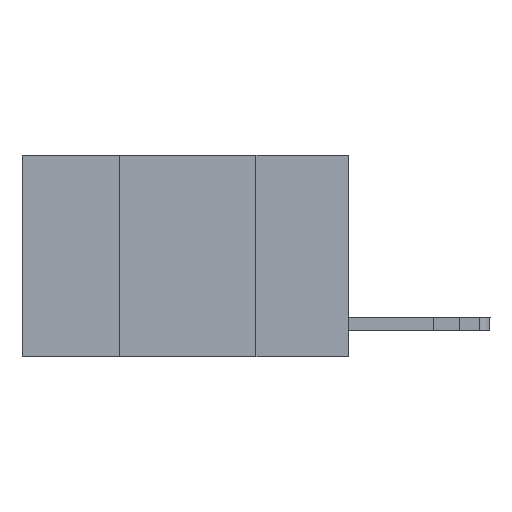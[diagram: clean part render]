
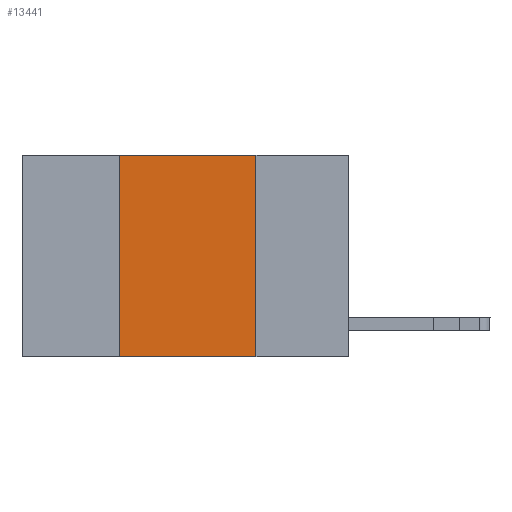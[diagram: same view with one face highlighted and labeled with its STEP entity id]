
A CAD part, left-side view. The second image highlights one B-rep face of the part: STEP entity #13441.
In plain terms, the highlighted planar face has unit normal (-1, 0, 0).
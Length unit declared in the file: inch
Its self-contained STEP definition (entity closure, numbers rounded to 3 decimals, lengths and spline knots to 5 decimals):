
#1074 = VECTOR ( 'NONE', #16984, 39.37008 ) ;
#1788 = CARTESIAN_POINT ( 'NONE',  ( 0., 0.17, -0.37 ) ) ;
#2278 = CARTESIAN_POINT ( 'NONE',  ( 0., 0.42, 0. ) ) ;
#3036 = VECTOR ( 'NONE', #17403, 39.37008 ) ;
#3111 = CARTESIAN_POINT ( 'NONE',  ( 0., 0.6, 0. ) ) ;
#3635 = VERTEX_POINT ( 'NONE', #1788 ) ;
#4269 = DIRECTION ( 'NONE',  ( 1., 0., 0. ) ) ;
#4271 = CARTESIAN_POINT ( 'NONE',  ( 0., 0.6, -0.37 ) ) ;
#5460 = VERTEX_POINT ( 'NONE', #18673 ) ;
#5673 = VERTEX_POINT ( 'NONE', #2278 ) ;
#6751 = CARTESIAN_POINT ( 'NONE',  ( 0., 0.17, 0. ) ) ;
#9118 = AXIS2_PLACEMENT_3D ( 'NONE', #11702, #4269, #17398 ) ;
#9364 = EDGE_CURVE ( 'NONE', #5673, #15221, #10644, .T. ) ;
#10622 = DIRECTION ( 'NONE',  ( 0., -1., 0. ) ) ;
#10644 = LINE ( 'NONE', #3111, #19452 ) ;
#10900 = ORIENTED_EDGE ( 'NONE', *, *, #15086, .F. ) ;
#10911 = CARTESIAN_POINT ( 'NONE',  ( 0., 0.17, 0. ) ) ;
#11702 = CARTESIAN_POINT ( 'NONE',  ( 0., 0.6, 0. ) ) ;
#12456 = LINE ( 'NONE', #6751, #21798 ) ;
#13012 = ORIENTED_EDGE ( 'NONE', *, *, #9364, .F. ) ;
#13257 = ORIENTED_EDGE ( 'NONE', *, *, #13972, .F. ) ;
#13441 = ADVANCED_FACE ( 'NONE', ( #22171 ), #19093, .F. ) ;
#13972 = EDGE_CURVE ( 'NONE', #5460, #5673, #16079, .T. ) ;
#15057 = ORIENTED_EDGE ( 'NONE', *, *, #23942, .T. ) ;
#15086 = EDGE_CURVE ( 'NONE', #15221, #3635, #12456, .T. ) ;
#15221 = VERTEX_POINT ( 'NONE', #10911 ) ;
#16079 = LINE ( 'NONE', #22542, #1074 ) ;
#16984 = DIRECTION ( 'NONE',  ( 0., 0., 1. ) ) ;
#17398 = DIRECTION ( 'NONE',  ( 0., 0., -1. ) ) ;
#17403 = DIRECTION ( 'NONE',  ( 0., -1., 0. ) ) ;
#17757 = EDGE_LOOP ( 'NONE', ( #10900, #13012, #13257, #15057 ) ) ;
#18673 = CARTESIAN_POINT ( 'NONE',  ( 0., 0.42, -0.37 ) ) ;
#19093 = PLANE ( 'NONE',  #9118 ) ;
#19452 = VECTOR ( 'NONE', #10622, 39.37008 ) ;
#21701 = DIRECTION ( 'NONE',  ( 0., 0., -1. ) ) ;
#21798 = VECTOR ( 'NONE', #21701, 39.37008 ) ;
#22171 = FACE_OUTER_BOUND ( 'NONE', #17757, .T. ) ;
#22339 = LINE ( 'NONE', #4271, #3036 ) ;
#22542 = CARTESIAN_POINT ( 'NONE',  ( 0., 0.42, 0. ) ) ;
#23942 = EDGE_CURVE ( 'NONE', #5460, #3635, #22339, .T. ) ;
